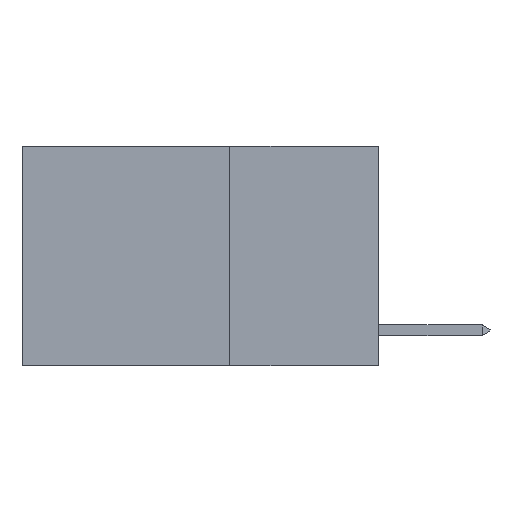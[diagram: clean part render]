
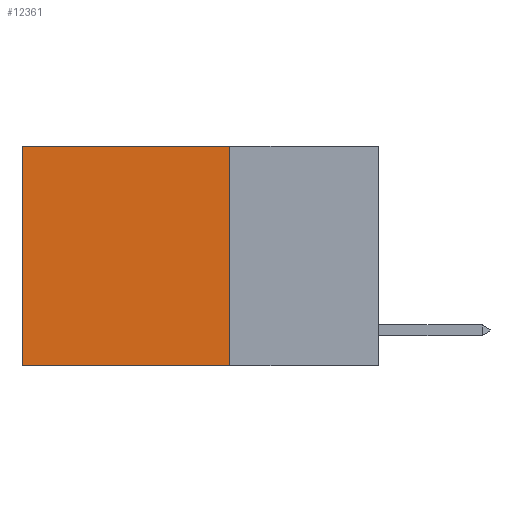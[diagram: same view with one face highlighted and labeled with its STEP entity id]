
A CAD part, left-side view. The second image highlights one B-rep face of the part: STEP entity #12361.
In plain terms, the highlighted planar face has unit normal (-1, 0, 0).
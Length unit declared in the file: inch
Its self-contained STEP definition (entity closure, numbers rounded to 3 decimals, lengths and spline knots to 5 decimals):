
#681 = EDGE_CURVE ( 'NONE', #14049, #2706, #7550, .T. ) ;
#1331 = VECTOR ( 'NONE', #8985, 39.37008 ) ;
#1548 = VERTEX_POINT ( 'NONE', #9845 ) ;
#1575 = CARTESIAN_POINT ( 'NONE',  ( 0.2625, 0.6, 0. ) ) ;
#1693 = EDGE_CURVE ( 'NONE', #13454, #1548, #5104, .T. ) ;
#2706 = VERTEX_POINT ( 'NONE', #6628 ) ;
#4473 = DIRECTION ( 'NONE',  ( 0., 0., -1. ) ) ;
#4722 = ORIENTED_EDGE ( 'NONE', *, *, #14866, .T. ) ;
#4838 = AXIS2_PLACEMENT_3D ( 'NONE', #10099, #12975, #4473 ) ;
#5030 = ORIENTED_EDGE ( 'NONE', *, *, #1693, .T. ) ;
#5089 = CARTESIAN_POINT ( 'NONE',  ( 0.2625, 0.25, 0. ) ) ;
#5104 = LINE ( 'NONE', #5089, #1331 ) ;
#6100 = LINE ( 'NONE', #1575, #10755 ) ;
#6628 = CARTESIAN_POINT ( 'NONE',  ( 0.2625, 0.6, -0.37 ) ) ;
#7550 = LINE ( 'NONE', #17929, #10871 ) ;
#8324 = CARTESIAN_POINT ( 'NONE',  ( 0.2625, 0.25, 0. ) ) ;
#8384 = CARTESIAN_POINT ( 'NONE',  ( 0.2625, 0.25, -0.37 ) ) ;
#8985 = DIRECTION ( 'NONE',  ( 0., 1., 0. ) ) ;
#9845 = CARTESIAN_POINT ( 'NONE',  ( 0.2625, 0.6, 0. ) ) ;
#10099 = CARTESIAN_POINT ( 'NONE',  ( 0.2625, 0.25, 0. ) ) ;
#10364 = FACE_OUTER_BOUND ( 'NONE', #16600, .T. ) ;
#10755 = VECTOR ( 'NONE', #14356, 39.37008 ) ;
#10871 = VECTOR ( 'NONE', #15024, 39.37008 ) ;
#12361 = ADVANCED_FACE ( 'NONE', ( #10364 ), #17178, .F. ) ;
#12625 = DIRECTION ( 'NONE',  ( 0., 0., -1. ) ) ;
#12975 = DIRECTION ( 'NONE',  ( 1., 0., 0. ) ) ;
#13127 = LINE ( 'NONE', #8324, #15155 ) ;
#13454 = VERTEX_POINT ( 'NONE', #15630 ) ;
#14049 = VERTEX_POINT ( 'NONE', #8384 ) ;
#14356 = DIRECTION ( 'NONE',  ( 0., 0., -1. ) ) ;
#14583 = ORIENTED_EDGE ( 'NONE', *, *, #681, .F. ) ;
#14660 = ORIENTED_EDGE ( 'NONE', *, *, #16682, .F. ) ;
#14866 = EDGE_CURVE ( 'NONE', #1548, #2706, #6100, .T. ) ;
#15024 = DIRECTION ( 'NONE',  ( 0., 1., 0. ) ) ;
#15155 = VECTOR ( 'NONE', #12625, 39.37008 ) ;
#15630 = CARTESIAN_POINT ( 'NONE',  ( 0.2625, 0.25, 0. ) ) ;
#16600 = EDGE_LOOP ( 'NONE', ( #4722, #14583, #14660, #5030 ) ) ;
#16682 = EDGE_CURVE ( 'NONE', #13454, #14049, #13127, .T. ) ;
#17178 = PLANE ( 'NONE',  #4838 ) ;
#17929 = CARTESIAN_POINT ( 'NONE',  ( 0.2625, 0.25, -0.37 ) ) ;
